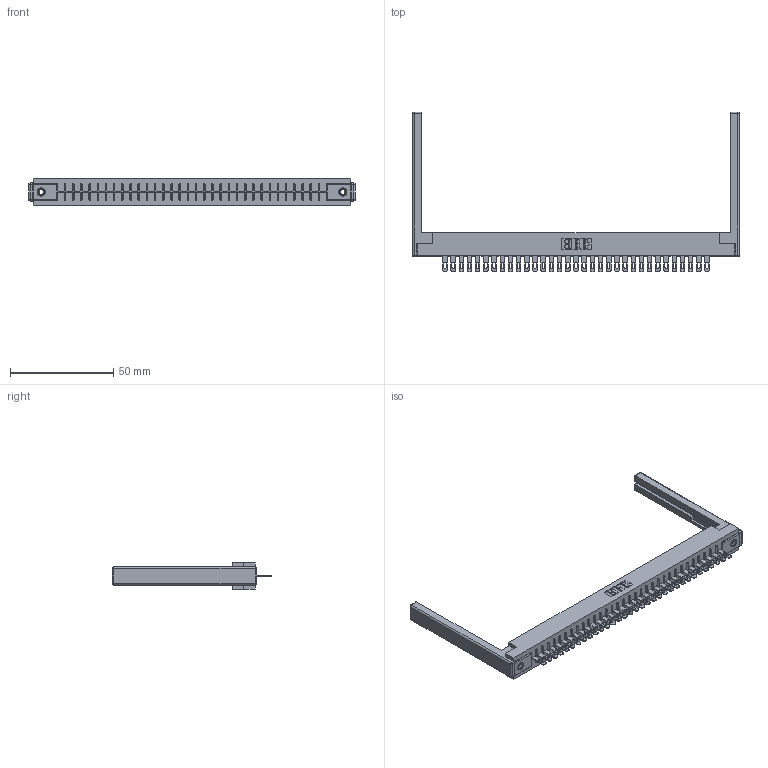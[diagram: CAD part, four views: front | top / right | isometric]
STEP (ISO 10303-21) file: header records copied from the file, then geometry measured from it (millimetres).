
FILE_DESCRIPTION (( 'STEP AP203' ), '1' );
FILE_NAME ('316-033-400-168.STEP', '2020-09-23T02:02:31', ( '' ), ( '' ), 'SwSTEP 2.0', 'SolidWorks 2020', '' );
FILE_SCHEMA (( 'CONFIG_CONTROL_DESIGN' ));
Length unit declared in the file: inch
Products named in the file (5): 306-290-001_100; 307-220-068; 306 Part_.156 Dia; 316-033-400-168; 345-250-001_345-250-001-102
Assembly tree (38 placements, depth 2):
  316-033-400-168
    306 Part_.156 Dia
    306-290-001_100  x33
    345-250-001_345-250-001-102  x2
    307-220-068  x2
Bounding box: 158.19 x 77.17 x 12.7 mm (x, y, z)
Volume: 21885.9 mm3; surface area: 22518.8 mm2
Topology: 38 solids, 38 shells, 2778 faces, 7801 edges, 5002 vertices
Faces by surface type: plane 1806, cylinder 816, sphere 140, cone 12, torus 4
Entity records: 34863 total; most frequent: CARTESIAN_POINT 5819, ORIENTED_EDGE 5760, DIRECTION 5752, EDGE_CURVE 2880, LINE 2242, VECTOR 2242, VERTEX_POINT 1822, AXIS2_PLACEMENT_3D 1755
